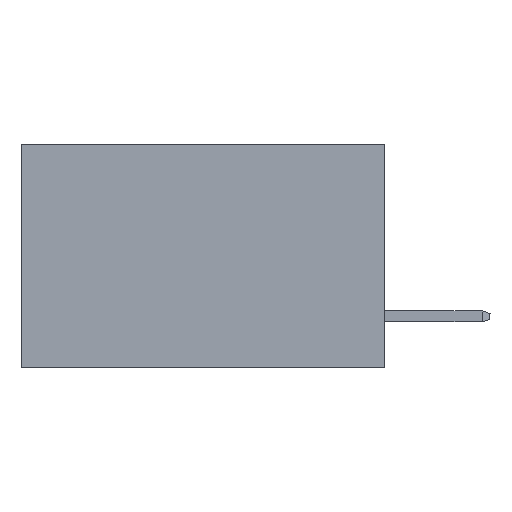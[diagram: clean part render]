
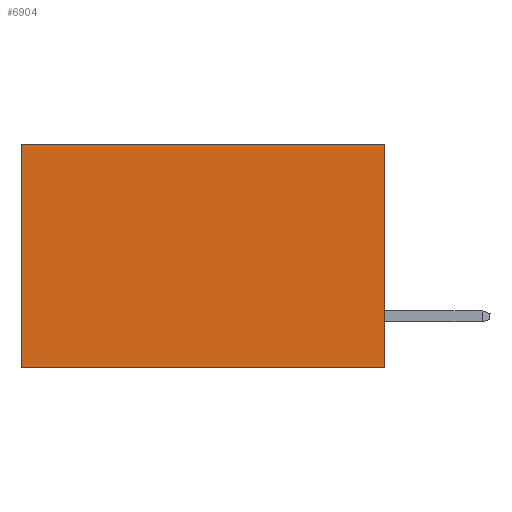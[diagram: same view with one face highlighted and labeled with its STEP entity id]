
A CAD part, left-side view. The second image highlights one B-rep face of the part: STEP entity #6904.
In plain terms, the highlighted planar face has unit normal (-1, 0, 0).
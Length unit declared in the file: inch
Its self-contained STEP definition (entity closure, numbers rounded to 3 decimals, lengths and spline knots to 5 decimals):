
#657 = CARTESIAN_POINT ( 'NONE',  ( 0.2615, 0., -0.37 ) ) ;
#767 = CARTESIAN_POINT ( 'NONE',  ( 0.2615, 0.6, 0. ) ) ;
#1044 = EDGE_CURVE ( 'NONE', #6228, #12455, #9028, .T. ) ;
#2374 = VECTOR ( 'NONE', #17218, 39.37008 ) ;
#3323 = EDGE_CURVE ( 'NONE', #12868, #14778, #11894, .T. ) ;
#3986 = DIRECTION ( 'NONE',  ( 0., 0., -1. ) ) ;
#4014 = ORIENTED_EDGE ( 'NONE', *, *, #9326, .T. ) ;
#4551 = AXIS2_PLACEMENT_3D ( 'NONE', #11485, #6669, #13066 ) ;
#4599 = CARTESIAN_POINT ( 'NONE',  ( 0.2615, 0., 0. ) ) ;
#4810 = CARTESIAN_POINT ( 'NONE',  ( 0.2615, 0., -0.37 ) ) ;
#6149 = PLANE ( 'NONE',  #4551 ) ;
#6228 = VERTEX_POINT ( 'NONE', #4599 ) ;
#6669 = DIRECTION ( 'NONE',  ( 1., 0., 0. ) ) ;
#6904 = ADVANCED_FACE ( 'NONE', ( #12787 ), #6149, .F. ) ;
#7251 = ORIENTED_EDGE ( 'NONE', *, *, #8387, .F. ) ;
#7714 = DIRECTION ( 'NONE',  ( 0., 1., 0. ) ) ;
#7906 = VECTOR ( 'NONE', #7714, 39.37008 ) ;
#8387 = EDGE_CURVE ( 'NONE', #6228, #12868, #16818, .T. ) ;
#9028 = LINE ( 'NONE', #13118, #7906 ) ;
#9326 = EDGE_CURVE ( 'NONE', #12455, #14778, #13170, .T. ) ;
#11238 = ORIENTED_EDGE ( 'NONE', *, *, #1044, .T. ) ;
#11485 = CARTESIAN_POINT ( 'NONE',  ( 0.2615, 0., -0.37 ) ) ;
#11894 = LINE ( 'NONE', #16996, #14865 ) ;
#12455 = VERTEX_POINT ( 'NONE', #767 ) ;
#12605 = CARTESIAN_POINT ( 'NONE',  ( 0.2615, 0.6, -0.37 ) ) ;
#12787 = FACE_OUTER_BOUND ( 'NONE', #12935, .T. ) ;
#12868 = VERTEX_POINT ( 'NONE', #657 ) ;
#12935 = EDGE_LOOP ( 'NONE', ( #4014, #14867, #7251, #11238 ) ) ;
#13066 = DIRECTION ( 'NONE',  ( 0., 0., -1. ) ) ;
#13118 = CARTESIAN_POINT ( 'NONE',  ( 0.2615, 0., 0. ) ) ;
#13170 = LINE ( 'NONE', #15833, #2374 ) ;
#14437 = DIRECTION ( 'NONE',  ( 0., 1., 0. ) ) ;
#14778 = VERTEX_POINT ( 'NONE', #12605 ) ;
#14865 = VECTOR ( 'NONE', #14437, 39.37008 ) ;
#14867 = ORIENTED_EDGE ( 'NONE', *, *, #3323, .F. ) ;
#15833 = CARTESIAN_POINT ( 'NONE',  ( 0.2615, 0.6, -0.37 ) ) ;
#16101 = VECTOR ( 'NONE', #3986, 39.37008 ) ;
#16818 = LINE ( 'NONE', #4810, #16101 ) ;
#16996 = CARTESIAN_POINT ( 'NONE',  ( 0.2615, 0., -0.37 ) ) ;
#17218 = DIRECTION ( 'NONE',  ( 0., 0., -1. ) ) ;
